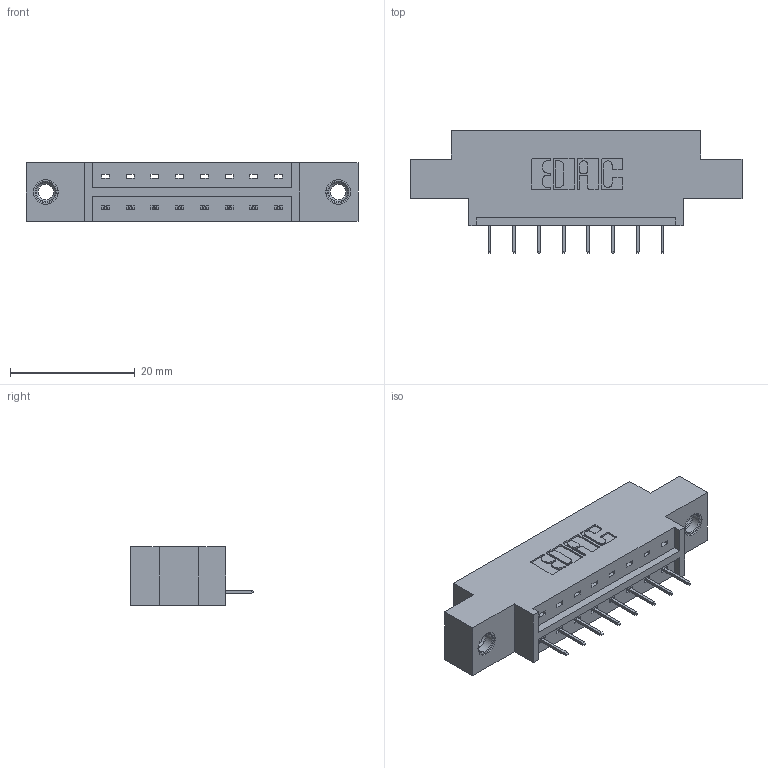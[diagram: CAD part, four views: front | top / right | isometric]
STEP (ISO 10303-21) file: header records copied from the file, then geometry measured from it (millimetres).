
FILE_DESCRIPTION (( 'STEP AP203' ), '1' );
FILE_NAME ('833-008-524-607.STEP', '2020-05-30T16:03:43', ( '' ), ( '' ), 'SwSTEP 2.0', 'SolidWorks 2020', '' );
FILE_SCHEMA (( 'CONFIG_CONTROL_DESIGN' ));
Length unit declared in the file: inch
Products named in the file (4): 833-008-524-607; 345-250-001_345-250-005-103; 345-292-001_345-293-124; 833 Part_Offset - .156 Dia - TI
Assembly tree (11 placements, depth 2):
  833-008-524-607
    833 Part_Offset - .156 Dia - TI
    345-292-001_345-293-124  x8
    345-250-001_345-250-005-103  x2
Bounding box: 53.24 x 19.69 x 9.4 mm (x, y, z)
Volume: 4792 mm3; surface area: 5089.2 mm2
Topology: 11 solids, 11 shells, 674 faces, 1899 edges, 1226 vertices
Faces by surface type: plane 490, cylinder 168, cone 12, torus 4
Entity records: 10680 total; most frequent: CARTESIAN_POINT 1829, ORIENTED_EDGE 1766, DIRECTION 1645, EDGE_CURVE 883, LINE 739, VECTOR 739, VERTEX_POINT 580, AXIS2_PLACEMENT_3D 453
